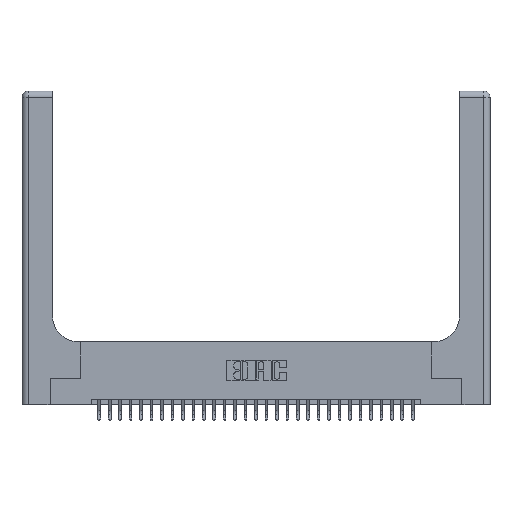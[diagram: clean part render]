
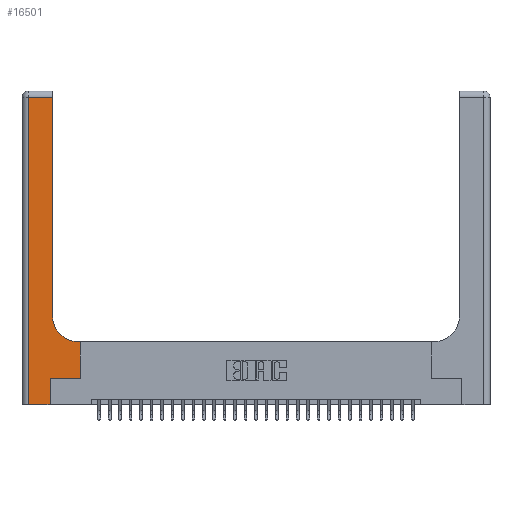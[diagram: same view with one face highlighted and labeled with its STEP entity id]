
A CAD part, top view. The second image highlights one B-rep face of the part: STEP entity #16501.
In plain terms, the highlighted planar face has unit normal (0, 0, 1).
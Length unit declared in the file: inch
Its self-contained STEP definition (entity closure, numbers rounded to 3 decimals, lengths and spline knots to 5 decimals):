
#184 = VERTEX_POINT ( 'NONE', #12568 ) ;
#458 = LINE ( 'NONE', #609, #20442 ) ;
#609 = CARTESIAN_POINT ( 'NONE',  ( 0.269, 0.25, 0.37 ) ) ;
#940 = PLANE ( 'NONE',  #7799 ) ;
#1308 = CARTESIAN_POINT ( 'NONE',  ( 0.5585, 0.6, 0.37 ) ) ;
#1922 = CARTESIAN_POINT ( 'NONE',  ( 0., 0., 0.37 ) ) ;
#4913 = DIRECTION ( 'NONE',  ( 0., 1., 0. ) ) ;
#5133 = VERTEX_POINT ( 'NONE', #14882 ) ;
#6064 = EDGE_CURVE ( 'NONE', #5133, #11450, #458, .T. ) ;
#6157 = EDGE_CURVE ( 'NONE', #184, #27096, #26881, .T. ) ;
#6267 = LINE ( 'NONE', #21520, #30420 ) ;
#6581 = LINE ( 'NONE', #11977, #15291 ) ;
#7129 = DIRECTION ( 'NONE',  ( 0., 1., 0. ) ) ;
#7779 = LINE ( 'NONE', #25012, #8525 ) ;
#7799 = AXIS2_PLACEMENT_3D ( 'NONE', #30357, #20646, #13170 ) ;
#7811 = LINE ( 'NONE', #1922, #10073 ) ;
#8049 = ORIENTED_EDGE ( 'NONE', *, *, #19366, .T. ) ;
#8274 = DIRECTION ( 'NONE',  ( 0., 0., -1. ) ) ;
#8525 = VECTOR ( 'NONE', #27852, 39.37008 ) ;
#9112 = DIRECTION ( 'NONE',  ( -1., 0., 0. ) ) ;
#9637 = ORIENTED_EDGE ( 'NONE', *, *, #6157, .T. ) ;
#10073 = VECTOR ( 'NONE', #21430, 39.37008 ) ;
#11107 = LINE ( 'NONE', #24026, #30385 ) ;
#11450 = VERTEX_POINT ( 'NONE', #17284 ) ;
#11977 = CARTESIAN_POINT ( 'NONE',  ( 0.269, 0., 0.37 ) ) ;
#12216 = LINE ( 'NONE', #23485, #16409 ) ;
#12568 = CARTESIAN_POINT ( 'NONE',  ( 0.5415, 0.6, 0.37 ) ) ;
#13170 = DIRECTION ( 'NONE',  ( -1., 0., 0. ) ) ;
#13348 = CARTESIAN_POINT ( 'NONE',  ( 0.5415, 0.85, 0.37 ) ) ;
#13951 = CARTESIAN_POINT ( 'NONE',  ( 0.269, 0., 0.37 ) ) ;
#14077 = EDGE_LOOP ( 'NONE', ( #24225, #25186, #23620, #15222, #25149, #23831, #29244, #8049, #9637 ) ) ;
#14080 = VERTEX_POINT ( 'NONE', #20163 ) ;
#14248 = DIRECTION ( 'NONE',  ( 0., -1., 0. ) ) ;
#14401 = EDGE_CURVE ( 'NONE', #14080, #23504, #6267, .T. ) ;
#14882 = CARTESIAN_POINT ( 'NONE',  ( 0.269, 0.25, 0.37 ) ) ;
#15222 = ORIENTED_EDGE ( 'NONE', *, *, #21220, .T. ) ;
#15291 = VECTOR ( 'NONE', #7129, 39.37008 ) ;
#16226 = DIRECTION ( 'NONE',  ( -1., 0., 0. ) ) ;
#16315 = CARTESIAN_POINT ( 'NONE',  ( 0.2915, 2.94, 0.37 ) ) ;
#16328 = CARTESIAN_POINT ( 'NONE',  ( 0.2915, 0.6, 0.37 ) ) ;
#16409 = VECTOR ( 'NONE', #9112, 39.37008 ) ;
#16501 = ADVANCED_FACE ( 'NONE', ( #29586 ), #940, .F. ) ;
#16593 = LINE ( 'NONE', #16328, #26777 ) ;
#17284 = CARTESIAN_POINT ( 'NONE',  ( 0.5585, 0.25, 0.37 ) ) ;
#18078 = VERTEX_POINT ( 'NONE', #1308 ) ;
#18534 = CARTESIAN_POINT ( 'NONE',  ( 0.06, 0., 0.37 ) ) ;
#18850 = CARTESIAN_POINT ( 'NONE',  ( 0.2915, 0.85, 0.37 ) ) ;
#19366 = EDGE_CURVE ( 'NONE', #18078, #184, #16593, .T. ) ;
#19899 = DIRECTION ( 'NONE',  ( 1., 0., 0. ) ) ;
#20163 = CARTESIAN_POINT ( 'NONE',  ( 0.06, 2.94, 0.37 ) ) ;
#20442 = VECTOR ( 'NONE', #19899, 39.37008 ) ;
#20641 = VERTEX_POINT ( 'NONE', #13951 ) ;
#20646 = DIRECTION ( 'NONE',  ( 0., 0., -1. ) ) ;
#21220 = EDGE_CURVE ( 'NONE', #23504, #20641, #7811, .T. ) ;
#21430 = DIRECTION ( 'NONE',  ( 1., 0., 0. ) ) ;
#21520 = CARTESIAN_POINT ( 'NONE',  ( 0.06, 3., 0.37 ) ) ;
#21635 = EDGE_CURVE ( 'NONE', #27096, #27548, #7779, .T. ) ;
#23485 = CARTESIAN_POINT ( 'NONE',  ( 0., 2.94, 0.37 ) ) ;
#23504 = VERTEX_POINT ( 'NONE', #18534 ) ;
#23592 = EDGE_CURVE ( 'NONE', #27548, #14080, #12216, .T. ) ;
#23620 = ORIENTED_EDGE ( 'NONE', *, *, #14401, .T. ) ;
#23831 = ORIENTED_EDGE ( 'NONE', *, *, #6064, .T. ) ;
#24026 = CARTESIAN_POINT ( 'NONE',  ( 0.5585, 0.25, 0.37 ) ) ;
#24225 = ORIENTED_EDGE ( 'NONE', *, *, #21635, .T. ) ;
#25012 = CARTESIAN_POINT ( 'NONE',  ( 0.2915, 3., 0.37 ) ) ;
#25149 = ORIENTED_EDGE ( 'NONE', *, *, #29122, .T. ) ;
#25186 = ORIENTED_EDGE ( 'NONE', *, *, #23592, .T. ) ;
#26389 = AXIS2_PLACEMENT_3D ( 'NONE', #13348, #8274, #27402 ) ;
#26777 = VECTOR ( 'NONE', #16226, 39.37008 ) ;
#26881 = CIRCLE ( 'NONE', #26389, 0.25 ) ;
#27096 = VERTEX_POINT ( 'NONE', #18850 ) ;
#27402 = DIRECTION ( 'NONE',  ( 1., 0., 0. ) ) ;
#27548 = VERTEX_POINT ( 'NONE', #16315 ) ;
#27852 = DIRECTION ( 'NONE',  ( 0., 1., 0. ) ) ;
#29093 = EDGE_CURVE ( 'NONE', #11450, #18078, #11107, .T. ) ;
#29122 = EDGE_CURVE ( 'NONE', #20641, #5133, #6581, .T. ) ;
#29244 = ORIENTED_EDGE ( 'NONE', *, *, #29093, .T. ) ;
#29586 = FACE_OUTER_BOUND ( 'NONE', #14077, .T. ) ;
#30357 = CARTESIAN_POINT ( 'NONE',  ( 0., 3., 0.37 ) ) ;
#30385 = VECTOR ( 'NONE', #4913, 39.37008 ) ;
#30420 = VECTOR ( 'NONE', #14248, 39.37008 ) ;
